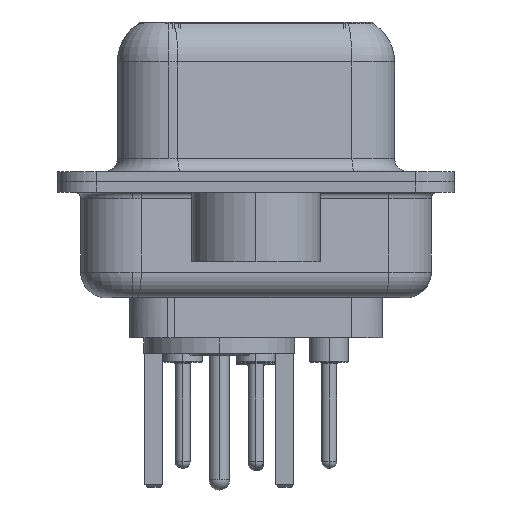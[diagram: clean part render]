
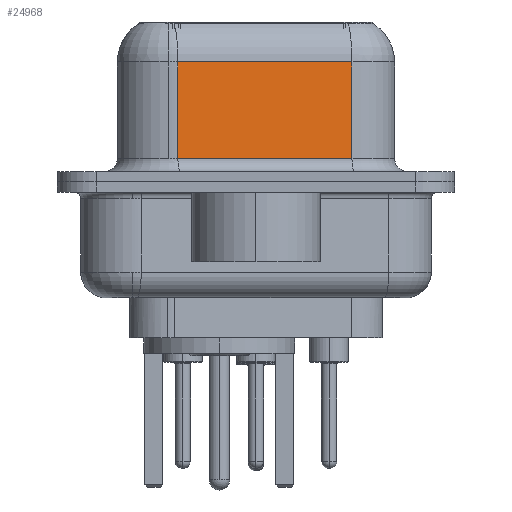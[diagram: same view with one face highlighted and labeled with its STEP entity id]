
A CAD part, left-side view. The second image highlights one B-rep face of the part: STEP entity #24968.
In plain terms, the highlighted planar face has unit normal (-0.985, -0.174, 0).
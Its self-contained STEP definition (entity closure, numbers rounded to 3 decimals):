
#297 = VECTOR ( 'NONE', #29598, 1000. ) ;
#1115 = VECTOR ( 'NONE', #33322, 1000. ) ;
#2094 = DIRECTION ( 'NONE',  ( -0.174, 0.985, 0. ) ) ;
#3646 = PLANE ( 'NONE',  #16880 ) ;
#4868 = ORIENTED_EDGE ( 'NONE', *, *, #5087, .T. ) ;
#5087 = EDGE_CURVE ( 'NONE', #28240, #15752, #6345, .T. ) ;
#5606 = FACE_OUTER_BOUND ( 'NONE', #5994, .T. ) ;
#5728 = CARTESIAN_POINT ( 'NONE',  ( 4.43, 3.028, 4.65 ) ) ;
#5994 = EDGE_LOOP ( 'NONE', ( #22142, #4868, #23835, #28722 ) ) ;
#6345 = LINE ( 'NONE', #25777, #26592 ) ;
#7729 = VERTEX_POINT ( 'NONE', #9027 ) ;
#7863 = VERTEX_POINT ( 'NONE', #9832 ) ;
#9027 = CARTESIAN_POINT ( 'NONE',  ( 5.621, -3.722, 0.9 ) ) ;
#9832 = CARTESIAN_POINT ( 'NONE',  ( 4.43, 3.028, 0.9 ) ) ;
#10494 = LINE ( 'NONE', #28118, #22890 ) ;
#13113 = LINE ( 'NONE', #18844, #297 ) ;
#15752 = VERTEX_POINT ( 'NONE', #5728 ) ;
#16880 = AXIS2_PLACEMENT_3D ( 'NONE', #19007, #27427, #30103 ) ;
#18623 = EDGE_CURVE ( 'NONE', #7863, #7729, #10494, .T. ) ;
#18844 = CARTESIAN_POINT ( 'NONE',  ( 4.43, 3.028, 6.4 ) ) ;
#19007 = CARTESIAN_POINT ( 'NONE',  ( 5.621, -3.722, 6.4 ) ) ;
#22142 = ORIENTED_EDGE ( 'NONE', *, *, #26952, .F. ) ;
#22890 = VECTOR ( 'NONE', #30894, 1000. ) ;
#23029 = EDGE_CURVE ( 'NONE', #15752, #7863, #13113, .T. ) ;
#23835 = ORIENTED_EDGE ( 'NONE', *, *, #23029, .T. ) ;
#24968 = ADVANCED_FACE ( 'NONE', ( #5606 ), #3646, .F. ) ;
#25405 = CARTESIAN_POINT ( 'NONE',  ( 5.621, -3.722, 6.4 ) ) ;
#25777 = CARTESIAN_POINT ( 'NONE',  ( 5.621, -3.722, 4.65 ) ) ;
#26592 = VECTOR ( 'NONE', #2094, 1000. ) ;
#26952 = EDGE_CURVE ( 'NONE', #28240, #7729, #27990, .T. ) ;
#27427 = DIRECTION ( 'NONE',  ( 0.985, 0.174, 0. ) ) ;
#27990 = LINE ( 'NONE', #25405, #1115 ) ;
#28118 = CARTESIAN_POINT ( 'NONE',  ( 5.621, -3.722, 0.9 ) ) ;
#28240 = VERTEX_POINT ( 'NONE', #28463 ) ;
#28463 = CARTESIAN_POINT ( 'NONE',  ( 5.621, -3.722, 4.65 ) ) ;
#28722 = ORIENTED_EDGE ( 'NONE', *, *, #18623, .T. ) ;
#29598 = DIRECTION ( 'NONE',  ( 0., 0., -1. ) ) ;
#30103 = DIRECTION ( 'NONE',  ( -0.174, 0.985, 0. ) ) ;
#30894 = DIRECTION ( 'NONE',  ( 0.174, -0.985, 0. ) ) ;
#33322 = DIRECTION ( 'NONE',  ( 0., 0., -1. ) ) ;
